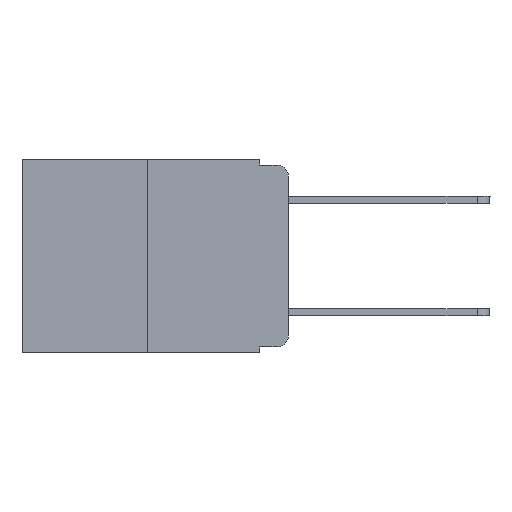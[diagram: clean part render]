
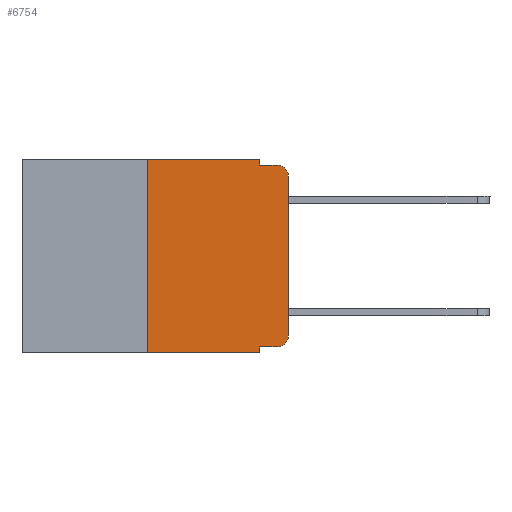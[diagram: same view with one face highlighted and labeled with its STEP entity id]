
A CAD part, left-side view. The second image highlights one B-rep face of the part: STEP entity #6754.
In plain terms, the highlighted planar face has unit normal (-1, 0, 0).
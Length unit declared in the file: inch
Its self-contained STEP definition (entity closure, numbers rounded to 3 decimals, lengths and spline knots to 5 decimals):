
#189 = LINE ( 'NONE', #2722, #10686 ) ;
#432 = DIRECTION ( 'NONE',  ( 0., -1., 0. ) ) ;
#490 = EDGE_CURVE ( 'NONE', #10355, #3998, #6865, .T. ) ;
#1222 = DIRECTION ( 'NONE',  ( -1., 0., 0. ) ) ;
#1565 = LINE ( 'NONE', #2692, #2013 ) ;
#1612 = CARTESIAN_POINT ( 'NONE',  ( 0., 0., -0.03 ) ) ;
#1935 = CARTESIAN_POINT ( 'NONE',  ( 0., 0.25, -0.343 ) ) ;
#1993 = ORIENTED_EDGE ( 'NONE', *, *, #8002, .T. ) ;
#1995 = VERTEX_POINT ( 'NONE', #13559 ) ;
#2013 = VECTOR ( 'NONE', #12456, 39.37008 ) ;
#2067 = DIRECTION ( 'NONE',  ( 0., -1., 0. ) ) ;
#2071 = DIRECTION ( 'NONE',  ( 0., 0., -1. ) ) ;
#2385 = ORIENTED_EDGE ( 'NONE', *, *, #3509, .F. ) ;
#2437 = VERTEX_POINT ( 'NONE', #2678 ) ;
#2678 = CARTESIAN_POINT ( 'NONE',  ( 0., 0.02, -0.333 ) ) ;
#2692 = CARTESIAN_POINT ( 'NONE',  ( 0., 0.25, 0. ) ) ;
#2722 = CARTESIAN_POINT ( 'NONE',  ( 0., 0.051, 0. ) ) ;
#2889 = DIRECTION ( 'NONE',  ( -1., 0., 0. ) ) ;
#3263 = CARTESIAN_POINT ( 'NONE',  ( 0., 0.473, -0.343 ) ) ;
#3333 = ORIENTED_EDGE ( 'NONE', *, *, #490, .F. ) ;
#3509 = EDGE_CURVE ( 'NONE', #4609, #9238, #8066, .T. ) ;
#3600 = ORIENTED_EDGE ( 'NONE', *, *, #11366, .F. ) ;
#3666 = ORIENTED_EDGE ( 'NONE', *, *, #6664, .T. ) ;
#3683 = DIRECTION ( 'NONE',  ( 0., 0., -1. ) ) ;
#3998 = VERTEX_POINT ( 'NONE', #12939 ) ;
#4022 = CARTESIAN_POINT ( 'NONE',  ( 0., 0., 0. ) ) ;
#4031 = AXIS2_PLACEMENT_3D ( 'NONE', #6669, #2889, #8874 ) ;
#4221 = ORIENTED_EDGE ( 'NONE', *, *, #7483, .F. ) ;
#4278 = CIRCLE ( 'NONE', #5792, 0.02 ) ;
#4471 = ORIENTED_EDGE ( 'NONE', *, *, #5099, .T. ) ;
#4609 = VERTEX_POINT ( 'NONE', #10793 ) ;
#4694 = ORIENTED_EDGE ( 'NONE', *, *, #6586, .T. ) ;
#5099 = EDGE_CURVE ( 'NONE', #2437, #1995, #4278, .T. ) ;
#5416 = VECTOR ( 'NONE', #2071, 39.37008 ) ;
#5583 = EDGE_LOOP ( 'NONE', ( #1993, #3666, #3333, #3600, #6414, #4221, #13453, #2385, #4694, #4471 ) ) ;
#5659 = VERTEX_POINT ( 'NONE', #1935 ) ;
#5792 = AXIS2_PLACEMENT_3D ( 'NONE', #6292, #1222, #7564 ) ;
#6292 = CARTESIAN_POINT ( 'NONE',  ( 0., 0.02, -0.313 ) ) ;
#6414 = ORIENTED_EDGE ( 'NONE', *, *, #14493, .F. ) ;
#6586 = EDGE_CURVE ( 'NONE', #4609, #2437, #7842, .T. ) ;
#6664 = EDGE_CURVE ( 'NONE', #7225, #3998, #12323, .T. ) ;
#6669 = CARTESIAN_POINT ( 'NONE',  ( 0., 0.02, -0.03 ) ) ;
#6754 = ADVANCED_FACE ( 'NONE', ( #9676 ), #8728, .F. ) ;
#6865 = LINE ( 'NONE', #11432, #7094 ) ;
#6896 = LINE ( 'NONE', #11696, #9244 ) ;
#7094 = VECTOR ( 'NONE', #15176, 39.37008 ) ;
#7225 = VERTEX_POINT ( 'NONE', #1612 ) ;
#7305 = DIRECTION ( 'NONE',  ( 1., 0., 0. ) ) ;
#7483 = EDGE_CURVE ( 'NONE', #5659, #11371, #1565, .T. ) ;
#7564 = DIRECTION ( 'NONE',  ( 0., 0., -1. ) ) ;
#7842 = LINE ( 'NONE', #12562, #11320 ) ;
#8002 = EDGE_CURVE ( 'NONE', #1995, #7225, #12357, .T. ) ;
#8066 = LINE ( 'NONE', #12873, #5416 ) ;
#8593 = VECTOR ( 'NONE', #8825, 39.37008 ) ;
#8728 = PLANE ( 'NONE',  #14815 ) ;
#8825 = DIRECTION ( 'NONE',  ( 0., 0., 1. ) ) ;
#8874 = DIRECTION ( 'NONE',  ( 0., 0., -1. ) ) ;
#9238 = VERTEX_POINT ( 'NONE', #14562 ) ;
#9244 = VECTOR ( 'NONE', #15358, 39.37008 ) ;
#9495 = CARTESIAN_POINT ( 'NONE',  ( 0., 0.051, -0.01 ) ) ;
#9676 = FACE_OUTER_BOUND ( 'NONE', #5583, .T. ) ;
#10318 = EDGE_CURVE ( 'NONE', #5659, #9238, #10532, .T. ) ;
#10355 = VERTEX_POINT ( 'NONE', #9495 ) ;
#10532 = LINE ( 'NONE', #3263, #10919 ) ;
#10686 = VECTOR ( 'NONE', #14588, 39.37008 ) ;
#10793 = CARTESIAN_POINT ( 'NONE',  ( 0., 0.051, -0.333 ) ) ;
#10919 = VECTOR ( 'NONE', #2067, 39.37008 ) ;
#11081 = CARTESIAN_POINT ( 'NONE',  ( 0., 0.25, 0. ) ) ;
#11320 = VECTOR ( 'NONE', #432, 39.37008 ) ;
#11366 = EDGE_CURVE ( 'NONE', #15097, #10355, #189, .T. ) ;
#11371 = VERTEX_POINT ( 'NONE', #11081 ) ;
#11432 = CARTESIAN_POINT ( 'NONE',  ( 0., 0.051, -0.01 ) ) ;
#11696 = CARTESIAN_POINT ( 'NONE',  ( 0., 0.473, 0. ) ) ;
#12129 = CARTESIAN_POINT ( 'NONE',  ( 0., 0.051, 0. ) ) ;
#12259 = CARTESIAN_POINT ( 'NONE',  ( 0., 0.473, 0. ) ) ;
#12323 = CIRCLE ( 'NONE', #4031, 0.02 ) ;
#12357 = LINE ( 'NONE', #4022, #8593 ) ;
#12456 = DIRECTION ( 'NONE',  ( 0., 0., 1. ) ) ;
#12562 = CARTESIAN_POINT ( 'NONE',  ( 0., 0.051, -0.333 ) ) ;
#12873 = CARTESIAN_POINT ( 'NONE',  ( 0., 0.051, 0. ) ) ;
#12939 = CARTESIAN_POINT ( 'NONE',  ( 0., 0.02, -0.01 ) ) ;
#13453 = ORIENTED_EDGE ( 'NONE', *, *, #10318, .T. ) ;
#13559 = CARTESIAN_POINT ( 'NONE',  ( 0., 0., -0.313 ) ) ;
#14493 = EDGE_CURVE ( 'NONE', #11371, #15097, #6896, .T. ) ;
#14562 = CARTESIAN_POINT ( 'NONE',  ( 0., 0.051, -0.343 ) ) ;
#14588 = DIRECTION ( 'NONE',  ( 0., 0., -1. ) ) ;
#14815 = AXIS2_PLACEMENT_3D ( 'NONE', #12259, #7305, #3683 ) ;
#15097 = VERTEX_POINT ( 'NONE', #12129 ) ;
#15176 = DIRECTION ( 'NONE',  ( 0., -1., 0. ) ) ;
#15358 = DIRECTION ( 'NONE',  ( 0., -1., 0. ) ) ;
